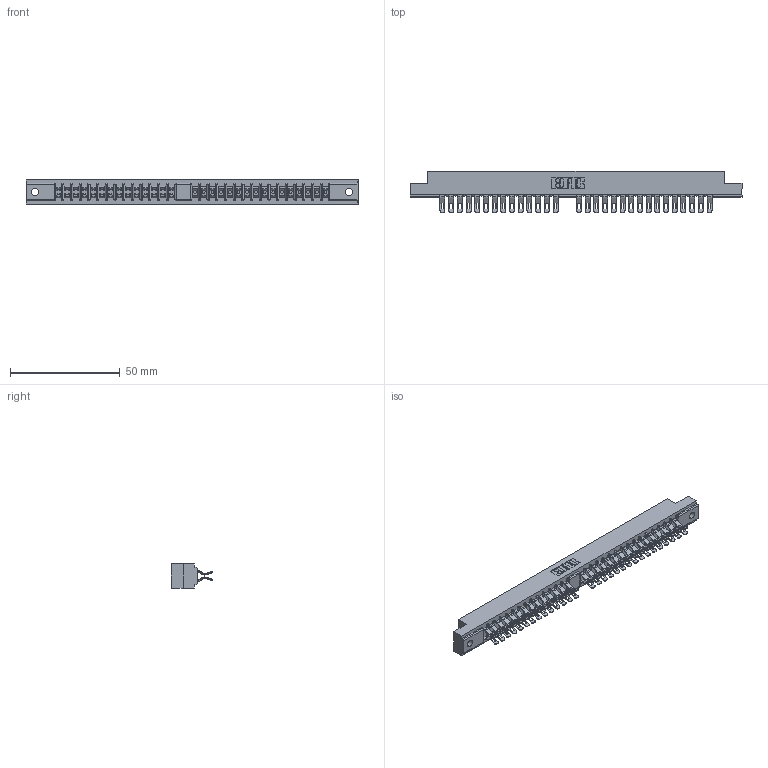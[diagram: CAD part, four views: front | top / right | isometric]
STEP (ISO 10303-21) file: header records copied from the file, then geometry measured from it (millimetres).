
FILE_DESCRIPTION (( 'STEP AP203' ), '1' );
FILE_NAME ('310-060-555-202.STEP', '2020-03-25T14:08:06', ( '' ), ( '' ), 'SwSTEP 2.0', 'SolidWorks 2016', '' );
FILE_SCHEMA (( 'CONFIG_CONTROL_DESIGN' ));
Length unit declared in the file: millimetre
Products named in the file (3): 310 Part_.128 Dia. Hole; 310-060-555-202; 307-290-001_555
Assembly tree (61 placements, depth 2):
  310-060-555-202
    310 Part_.128 Dia. Hole
    307-290-001_555  x60
Bounding box: 151.21 x 18.69 x 10.97 mm (x, y, z)
Volume: 13152.5 mm3; surface area: 18671.9 mm2
Topology: 61 solids, 61 shells, 3826 faces, 11221 edges, 7310 vertices
Faces by surface type: plane 2124, cylinder 1638, sphere 64
Entity records: 29123 total; most frequent: CARTESIAN_POINT 4775, ORIENTED_EDGE 4732, DIRECTION 4690, EDGE_CURVE 2366, LINE 1804, VECTOR 1804, VERTEX_POINT 1528, AXIS2_PLACEMENT_3D 1443
